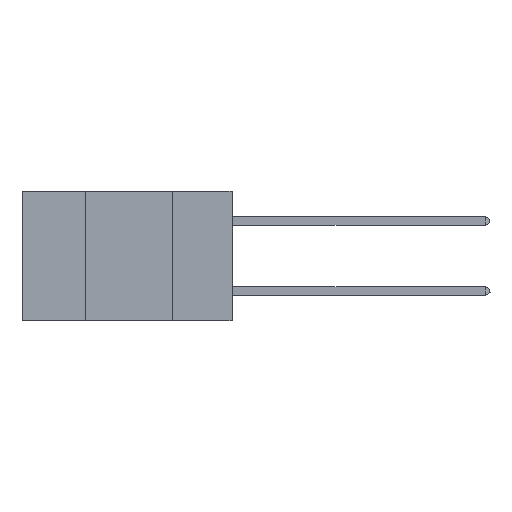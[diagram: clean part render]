
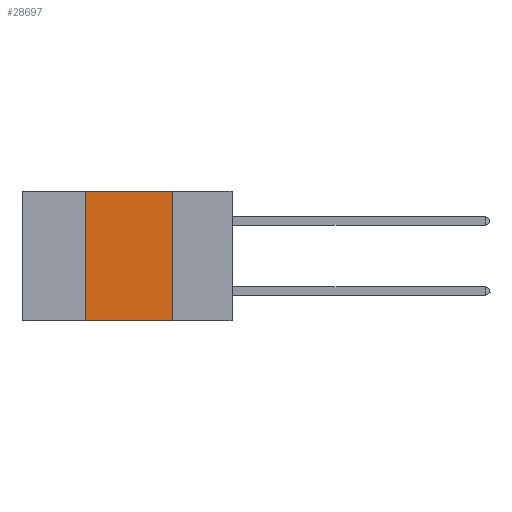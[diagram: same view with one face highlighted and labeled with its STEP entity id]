
A CAD part, left-side view. The second image highlights one B-rep face of the part: STEP entity #28697.
In plain terms, the highlighted planar face has unit normal (-1, 0, 0).
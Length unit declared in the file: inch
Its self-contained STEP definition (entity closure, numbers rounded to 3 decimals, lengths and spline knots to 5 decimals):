
#1357 = EDGE_CURVE ( 'NONE', #29266, #15197, #16351, .T. ) ;
#2287 = VECTOR ( 'NONE', #20331, 39.37008 ) ;
#2619 = CARTESIAN_POINT ( 'NONE',  ( 0., 0.6, 0. ) ) ;
#2875 = CARTESIAN_POINT ( 'NONE',  ( 0., 0.17, 0. ) ) ;
#3704 = CARTESIAN_POINT ( 'NONE',  ( 0., 0.42, 0. ) ) ;
#4098 = FACE_OUTER_BOUND ( 'NONE', #11938, .T. ) ;
#5429 = CARTESIAN_POINT ( 'NONE',  ( 0., 0.17, -0.37 ) ) ;
#6074 = PLANE ( 'NONE',  #21078 ) ;
#6595 = LINE ( 'NONE', #3704, #22657 ) ;
#9721 = VECTOR ( 'NONE', #16669, 39.37008 ) ;
#9873 = DIRECTION ( 'NONE',  ( 1., 0., 0. ) ) ;
#10154 = CARTESIAN_POINT ( 'NONE',  ( 0., 0.17, 0. ) ) ;
#10596 = ORIENTED_EDGE ( 'NONE', *, *, #19116, .F. ) ;
#11832 = CARTESIAN_POINT ( 'NONE',  ( 0., 0.6, -0.37 ) ) ;
#11938 = EDGE_LOOP ( 'NONE', ( #28621, #10596, #25443, #13102 ) ) ;
#12112 = LINE ( 'NONE', #2619, #19522 ) ;
#13102 = ORIENTED_EDGE ( 'NONE', *, *, #19984, .T. ) ;
#14310 = VERTEX_POINT ( 'NONE', #31363 ) ;
#14412 = DIRECTION ( 'NONE',  ( 0., 0., 1. ) ) ;
#15197 = VERTEX_POINT ( 'NONE', #5429 ) ;
#15266 = DIRECTION ( 'NONE',  ( 0., -1., 0. ) ) ;
#16351 = LINE ( 'NONE', #2875, #2287 ) ;
#16669 = DIRECTION ( 'NONE',  ( 0., -1., 0. ) ) ;
#19116 = EDGE_CURVE ( 'NONE', #14310, #29266, #12112, .T. ) ;
#19515 = CARTESIAN_POINT ( 'NONE',  ( 0., 0.42, -0.37 ) ) ;
#19522 = VECTOR ( 'NONE', #15266, 39.37008 ) ;
#19537 = DIRECTION ( 'NONE',  ( 0., 0., -1. ) ) ;
#19713 = EDGE_CURVE ( 'NONE', #31659, #14310, #6595, .T. ) ;
#19984 = EDGE_CURVE ( 'NONE', #31659, #15197, #22632, .T. ) ;
#20331 = DIRECTION ( 'NONE',  ( 0., 0., -1. ) ) ;
#21078 = AXIS2_PLACEMENT_3D ( 'NONE', #24327, #9873, #19537 ) ;
#22632 = LINE ( 'NONE', #11832, #9721 ) ;
#22657 = VECTOR ( 'NONE', #14412, 39.37008 ) ;
#24327 = CARTESIAN_POINT ( 'NONE',  ( 0., 0.6, 0. ) ) ;
#25443 = ORIENTED_EDGE ( 'NONE', *, *, #19713, .F. ) ;
#28621 = ORIENTED_EDGE ( 'NONE', *, *, #1357, .F. ) ;
#28697 = ADVANCED_FACE ( 'NONE', ( #4098 ), #6074, .F. ) ;
#29266 = VERTEX_POINT ( 'NONE', #10154 ) ;
#31363 = CARTESIAN_POINT ( 'NONE',  ( 0., 0.42, 0. ) ) ;
#31659 = VERTEX_POINT ( 'NONE', #19515 ) ;
